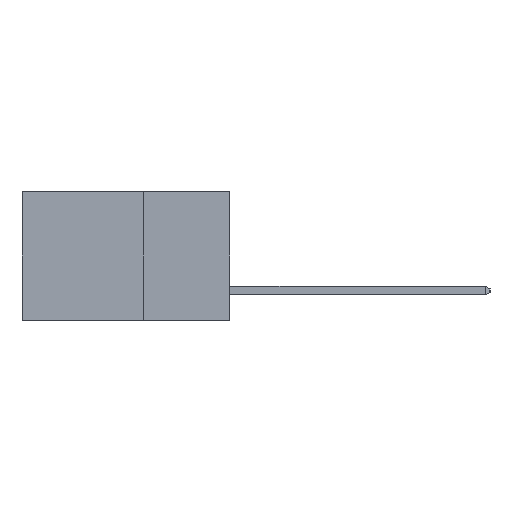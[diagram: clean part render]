
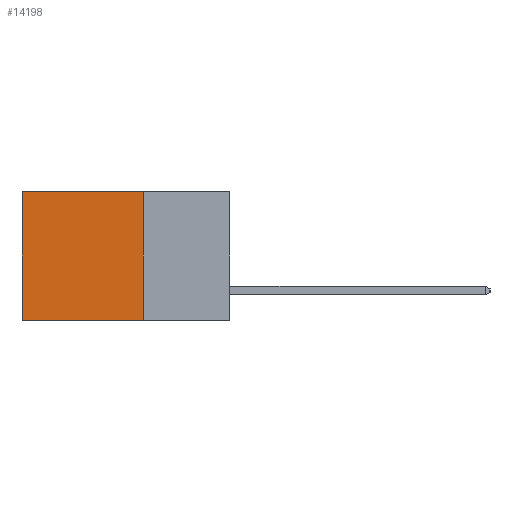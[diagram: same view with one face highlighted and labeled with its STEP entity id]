
A CAD part, left-side view. The second image highlights one B-rep face of the part: STEP entity #14198.
In plain terms, the highlighted planar face has unit normal (-1, 0, 0).
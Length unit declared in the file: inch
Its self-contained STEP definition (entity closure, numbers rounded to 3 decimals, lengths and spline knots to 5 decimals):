
#212 = EDGE_CURVE ( 'NONE', #1504, #16023, #14435, .T. ) ;
#830 = CARTESIAN_POINT ( 'NONE',  ( 0.298, 0.6, 0. ) ) ;
#897 = EDGE_LOOP ( 'NONE', ( #13300, #11139, #10785, #12373 ) ) ;
#1504 = VERTEX_POINT ( 'NONE', #12697 ) ;
#2257 = VERTEX_POINT ( 'NONE', #9791 ) ;
#2301 = FACE_OUTER_BOUND ( 'NONE', #897, .T. ) ;
#3583 = DIRECTION ( 'NONE',  ( 1., 0., 0. ) ) ;
#3637 = EDGE_CURVE ( 'NONE', #13111, #2257, #5664, .T. ) ;
#4730 = LINE ( 'NONE', #5331, #11434 ) ;
#4753 = EDGE_CURVE ( 'NONE', #1504, #13111, #5431, .T. ) ;
#5021 = VECTOR ( 'NONE', #7327, 39.37008 ) ;
#5293 = DIRECTION ( 'NONE',  ( 0., 0., -1. ) ) ;
#5331 = CARTESIAN_POINT ( 'NONE',  ( 0.298, 0.6, 0. ) ) ;
#5431 = LINE ( 'NONE', #8587, #5021 ) ;
#5664 = LINE ( 'NONE', #9284, #11933 ) ;
#7327 = DIRECTION ( 'NONE',  ( 0., 0., -1. ) ) ;
#7764 = EDGE_CURVE ( 'NONE', #16023, #2257, #4730, .T. ) ;
#8587 = CARTESIAN_POINT ( 'NONE',  ( 0.298, 0.25, 0. ) ) ;
#8670 = PLANE ( 'NONE',  #9333 ) ;
#9068 = CARTESIAN_POINT ( 'NONE',  ( 0.298, 0.25, -0.37 ) ) ;
#9284 = CARTESIAN_POINT ( 'NONE',  ( 0.298, 0.25, -0.37 ) ) ;
#9333 = AXIS2_PLACEMENT_3D ( 'NONE', #11142, #3583, #12414 ) ;
#9791 = CARTESIAN_POINT ( 'NONE',  ( 0.298, 0.6, -0.37 ) ) ;
#10501 = DIRECTION ( 'NONE',  ( 0., 1., 0. ) ) ;
#10785 = ORIENTED_EDGE ( 'NONE', *, *, #4753, .F. ) ;
#11139 = ORIENTED_EDGE ( 'NONE', *, *, #3637, .F. ) ;
#11142 = CARTESIAN_POINT ( 'NONE',  ( 0.298, 0.25, 0. ) ) ;
#11434 = VECTOR ( 'NONE', #5293, 39.37008 ) ;
#11933 = VECTOR ( 'NONE', #10501, 39.37008 ) ;
#12373 = ORIENTED_EDGE ( 'NONE', *, *, #212, .T. ) ;
#12414 = DIRECTION ( 'NONE',  ( 0., 0., -1. ) ) ;
#12697 = CARTESIAN_POINT ( 'NONE',  ( 0.298, 0.25, 0. ) ) ;
#13092 = DIRECTION ( 'NONE',  ( 0., 1., 0. ) ) ;
#13111 = VERTEX_POINT ( 'NONE', #9068 ) ;
#13300 = ORIENTED_EDGE ( 'NONE', *, *, #7764, .T. ) ;
#14060 = VECTOR ( 'NONE', #13092, 39.37008 ) ;
#14198 = ADVANCED_FACE ( 'NONE', ( #2301 ), #8670, .F. ) ;
#14435 = LINE ( 'NONE', #14733, #14060 ) ;
#14733 = CARTESIAN_POINT ( 'NONE',  ( 0.298, 0.25, 0. ) ) ;
#16023 = VERTEX_POINT ( 'NONE', #830 ) ;
